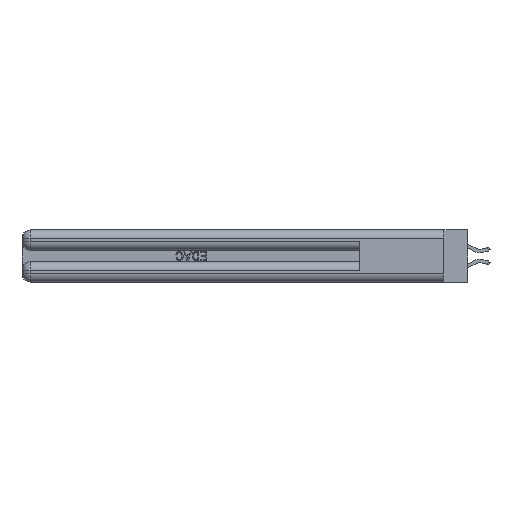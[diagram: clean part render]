
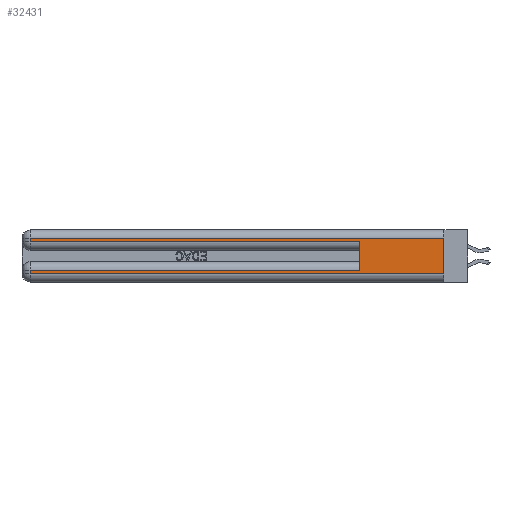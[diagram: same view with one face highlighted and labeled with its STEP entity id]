
A CAD part, left-side view. The second image highlights one B-rep face of the part: STEP entity #32431.
In plain terms, the highlighted planar face has unit normal (-1, 0, 0).
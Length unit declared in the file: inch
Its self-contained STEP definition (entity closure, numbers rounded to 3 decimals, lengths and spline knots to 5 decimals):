
#393 = CARTESIAN_POINT ( 'NONE',  ( 0., 0., 0.37 ) ) ;
#553 = LINE ( 'NONE', #3787, #21656 ) ;
#825 = DIRECTION ( 'NONE',  ( 1., 0., 0. ) ) ;
#1192 = LINE ( 'NONE', #39125, #18003 ) ;
#2023 = AXIS2_PLACEMENT_3D ( 'NONE', #393, #825, #31074 ) ;
#2871 = VECTOR ( 'NONE', #8816, 39.37008 ) ;
#3787 = CARTESIAN_POINT ( 'NONE',  ( 0., 0., 0.085 ) ) ;
#3819 = CARTESIAN_POINT ( 'NONE',  ( 0., 2.94, 0.37 ) ) ;
#5127 = LINE ( 'NONE', #3819, #39997 ) ;
#5219 = EDGE_CURVE ( 'NONE', #12385, #23478, #42978, .T. ) ;
#5580 = CARTESIAN_POINT ( 'NONE',  ( 0., 0., 0.31 ) ) ;
#6175 = EDGE_CURVE ( 'NONE', #36911, #12922, #553, .T. ) ;
#7292 = PLANE ( 'NONE',  #2023 ) ;
#7658 = EDGE_CURVE ( 'NONE', #34389, #33582, #30567, .T. ) ;
#8816 = DIRECTION ( 'NONE',  ( 0., 0., -1. ) ) ;
#10265 = CARTESIAN_POINT ( 'NONE',  ( 0., 2.94, 0.31 ) ) ;
#10699 = CARTESIAN_POINT ( 'NONE',  ( 0., 0., 0.37 ) ) ;
#12385 = VERTEX_POINT ( 'NONE', #35649 ) ;
#12922 = VERTEX_POINT ( 'NONE', #38646 ) ;
#14425 = ORIENTED_EDGE ( 'NONE', *, *, #7658, .T. ) ;
#15249 = DIRECTION ( 'NONE',  ( 0., 0., 1. ) ) ;
#17565 = CARTESIAN_POINT ( 'NONE',  ( 0., 0.6, 0.145 ) ) ;
#18003 = VECTOR ( 'NONE', #28934, 39.37008 ) ;
#19185 = CARTESIAN_POINT ( 'NONE',  ( 0., 0., 0.06 ) ) ;
#21279 = ORIENTED_EDGE ( 'NONE', *, *, #41349, .F. ) ;
#21513 = ORIENTED_EDGE ( 'NONE', *, *, #42395, .F. ) ;
#21656 = VECTOR ( 'NONE', #35062, 39.37008 ) ;
#22380 = CARTESIAN_POINT ( 'NONE',  ( 0., 0., 0.06 ) ) ;
#23478 = VERTEX_POINT ( 'NONE', #19185 ) ;
#23535 = EDGE_CURVE ( 'NONE', #12922, #12385, #40852, .T. ) ;
#24130 = DIRECTION ( 'NONE',  ( 0., 0., -1. ) ) ;
#26560 = LINE ( 'NONE', #10699, #33482 ) ;
#26898 = LINE ( 'NONE', #17565, #35902 ) ;
#28161 = ORIENTED_EDGE ( 'NONE', *, *, #6175, .T. ) ;
#28643 = EDGE_CURVE ( 'NONE', #33582, #38959, #5127, .T. ) ;
#28934 = DIRECTION ( 'NONE',  ( 0., -1., 0. ) ) ;
#29958 = CARTESIAN_POINT ( 'NONE',  ( 0., 0.6, 0.285 ) ) ;
#30567 = LINE ( 'NONE', #5580, #33232 ) ;
#30976 = ORIENTED_EDGE ( 'NONE', *, *, #42652, .T. ) ;
#31074 = DIRECTION ( 'NONE',  ( 0., 0., -1. ) ) ;
#31121 = DIRECTION ( 'NONE',  ( 0., 0., -1. ) ) ;
#31293 = CARTESIAN_POINT ( 'NONE',  ( 0., 0., 0.31 ) ) ;
#32431 = ADVANCED_FACE ( 'NONE', ( #40871 ), #7292, .F. ) ;
#32461 = ORIENTED_EDGE ( 'NONE', *, *, #28643, .T. ) ;
#32608 = DIRECTION ( 'NONE',  ( 0., 1., 0. ) ) ;
#33232 = VECTOR ( 'NONE', #32608, 39.37008 ) ;
#33482 = VECTOR ( 'NONE', #31121, 39.37008 ) ;
#33582 = VERTEX_POINT ( 'NONE', #10265 ) ;
#34389 = VERTEX_POINT ( 'NONE', #31293 ) ;
#34753 = VERTEX_POINT ( 'NONE', #29958 ) ;
#35062 = DIRECTION ( 'NONE',  ( 0., 1., 0. ) ) ;
#35649 = CARTESIAN_POINT ( 'NONE',  ( 0., 2.94, 0.06 ) ) ;
#35902 = VECTOR ( 'NONE', #15249, 39.37008 ) ;
#36911 = VERTEX_POINT ( 'NONE', #37381 ) ;
#37381 = CARTESIAN_POINT ( 'NONE',  ( 0., 0.6, 0.085 ) ) ;
#38462 = EDGE_LOOP ( 'NONE', ( #21513, #14425, #32461, #30976, #21279, #28161, #42486, #39922 ) ) ;
#38646 = CARTESIAN_POINT ( 'NONE',  ( 0., 2.94, 0.085 ) ) ;
#38959 = VERTEX_POINT ( 'NONE', #42167 ) ;
#39125 = CARTESIAN_POINT ( 'NONE',  ( 0., 0., 0.285 ) ) ;
#39922 = ORIENTED_EDGE ( 'NONE', *, *, #5219, .T. ) ;
#39997 = VECTOR ( 'NONE', #24130, 39.37008 ) ;
#40146 = DIRECTION ( 'NONE',  ( 0., -1., 0. ) ) ;
#40852 = LINE ( 'NONE', #42418, #2871 ) ;
#40871 = FACE_OUTER_BOUND ( 'NONE', #38462, .T. ) ;
#41349 = EDGE_CURVE ( 'NONE', #36911, #34753, #26898, .T. ) ;
#41887 = VECTOR ( 'NONE', #40146, 39.37008 ) ;
#42167 = CARTESIAN_POINT ( 'NONE',  ( 0., 2.94, 0.285 ) ) ;
#42395 = EDGE_CURVE ( 'NONE', #34389, #23478, #26560, .T. ) ;
#42418 = CARTESIAN_POINT ( 'NONE',  ( 0., 2.94, 0.37 ) ) ;
#42486 = ORIENTED_EDGE ( 'NONE', *, *, #23535, .T. ) ;
#42652 = EDGE_CURVE ( 'NONE', #38959, #34753, #1192, .T. ) ;
#42978 = LINE ( 'NONE', #22380, #41887 ) ;
